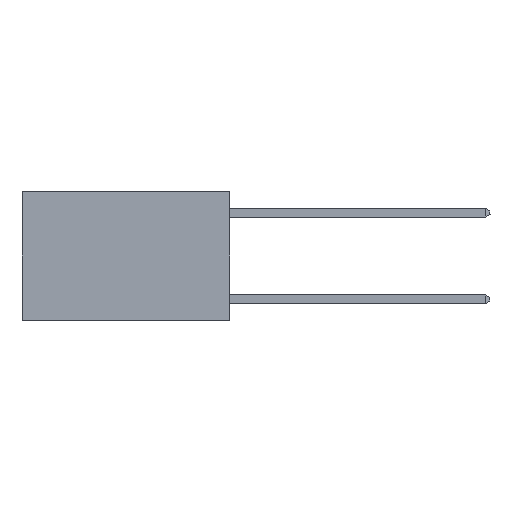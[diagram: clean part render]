
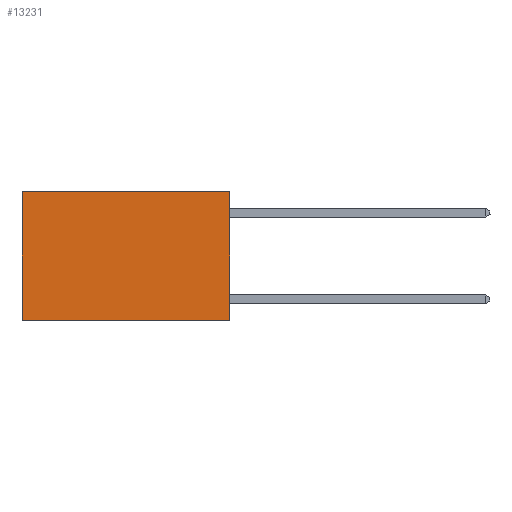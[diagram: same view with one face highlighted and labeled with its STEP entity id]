
A CAD part, left-side view. The second image highlights one B-rep face of the part: STEP entity #13231.
In plain terms, the highlighted planar face has unit normal (-1, 0, 0).
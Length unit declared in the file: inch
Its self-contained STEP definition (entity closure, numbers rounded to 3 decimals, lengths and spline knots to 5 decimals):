
#395 = CARTESIAN_POINT ( 'NONE',  ( 0.2625, 0.6, 0. ) ) ;
#741 = LINE ( 'NONE', #2124, #11999 ) ;
#910 = EDGE_CURVE ( 'NONE', #16114, #3319, #15254, .T. ) ;
#1439 = CARTESIAN_POINT ( 'NONE',  ( 0.2625, 0.6, 0. ) ) ;
#2100 = EDGE_CURVE ( 'NONE', #2574, #2872, #741, .T. ) ;
#2124 = CARTESIAN_POINT ( 'NONE',  ( 0.2625, 0., 0. ) ) ;
#2419 = EDGE_CURVE ( 'NONE', #2872, #3319, #11571, .T. ) ;
#2574 = VERTEX_POINT ( 'NONE', #4418 ) ;
#2687 = DIRECTION ( 'NONE',  ( 0., 0., -1. ) ) ;
#2872 = VERTEX_POINT ( 'NONE', #1439 ) ;
#2932 = VECTOR ( 'NONE', #2687, 39.37008 ) ;
#3319 = VERTEX_POINT ( 'NONE', #4284 ) ;
#4284 = CARTESIAN_POINT ( 'NONE',  ( 0.2625, 0.6, -0.37 ) ) ;
#4324 = VECTOR ( 'NONE', #16121, 39.37008 ) ;
#4418 = CARTESIAN_POINT ( 'NONE',  ( 0.2625, 0., 0. ) ) ;
#4870 = FACE_OUTER_BOUND ( 'NONE', #8505, .T. ) ;
#6344 = CARTESIAN_POINT ( 'NONE',  ( 0.2625, 0., 0. ) ) ;
#6606 = CARTESIAN_POINT ( 'NONE',  ( 0.2625, 0., -0.37 ) ) ;
#7244 = ORIENTED_EDGE ( 'NONE', *, *, #2100, .T. ) ;
#7662 = VECTOR ( 'NONE', #12599, 39.37008 ) ;
#8505 = EDGE_LOOP ( 'NONE', ( #16149, #14421, #9726, #7244 ) ) ;
#9231 = EDGE_CURVE ( 'NONE', #2574, #16114, #13624, .T. ) ;
#9726 = ORIENTED_EDGE ( 'NONE', *, *, #9231, .F. ) ;
#9761 = CARTESIAN_POINT ( 'NONE',  ( 0.2625, 0., 0. ) ) ;
#11098 = DIRECTION ( 'NONE',  ( 1., 0., 0. ) ) ;
#11334 = DIRECTION ( 'NONE',  ( 0., 0., -1. ) ) ;
#11571 = LINE ( 'NONE', #395, #2932 ) ;
#11999 = VECTOR ( 'NONE', #14480, 39.37008 ) ;
#12599 = DIRECTION ( 'NONE',  ( 0., 1., 0. ) ) ;
#13231 = ADVANCED_FACE ( 'NONE', ( #4870 ), #13748, .F. ) ;
#13624 = LINE ( 'NONE', #9761, #4324 ) ;
#13748 = PLANE ( 'NONE',  #14271 ) ;
#14271 = AXIS2_PLACEMENT_3D ( 'NONE', #6344, #11098, #11334 ) ;
#14328 = CARTESIAN_POINT ( 'NONE',  ( 0.2625, 0., -0.37 ) ) ;
#14421 = ORIENTED_EDGE ( 'NONE', *, *, #910, .F. ) ;
#14480 = DIRECTION ( 'NONE',  ( 0., 1., 0. ) ) ;
#15254 = LINE ( 'NONE', #6606, #7662 ) ;
#16114 = VERTEX_POINT ( 'NONE', #14328 ) ;
#16121 = DIRECTION ( 'NONE',  ( 0., 0., -1. ) ) ;
#16149 = ORIENTED_EDGE ( 'NONE', *, *, #2419, .T. ) ;
